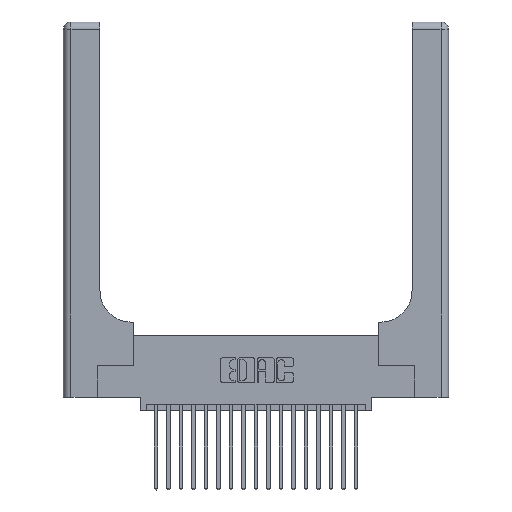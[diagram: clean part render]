
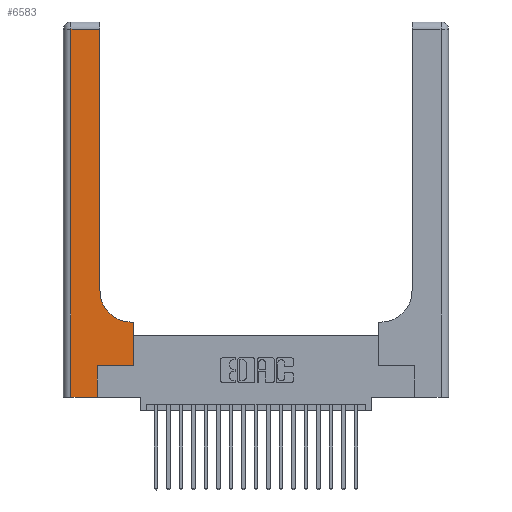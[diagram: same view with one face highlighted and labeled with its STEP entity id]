
A CAD part, top view. The second image highlights one B-rep face of the part: STEP entity #6583.
In plain terms, the highlighted planar face has unit normal (0, 0, 1).
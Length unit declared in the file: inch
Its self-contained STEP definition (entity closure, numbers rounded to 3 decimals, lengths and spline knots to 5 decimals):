
#160 = CARTESIAN_POINT ( 'NONE',  ( 0.06, 2.94, 0.37 ) ) ;
#549 = CARTESIAN_POINT ( 'NONE',  ( 0., 0., 0.37 ) ) ;
#964 = DIRECTION ( 'NONE',  ( 1., 0., 0. ) ) ;
#1575 = LINE ( 'NONE', #14638, #7964 ) ;
#1831 = VERTEX_POINT ( 'NONE', #12233 ) ;
#1888 = LINE ( 'NONE', #549, #21848 ) ;
#2194 = DIRECTION ( 'NONE',  ( 1., 0., 0. ) ) ;
#2305 = DIRECTION ( 'NONE',  ( 0., 1., 0. ) ) ;
#2744 = CARTESIAN_POINT ( 'NONE',  ( 0.5415, 0.85, 0.37 ) ) ;
#3574 = VERTEX_POINT ( 'NONE', #21102 ) ;
#3605 = EDGE_CURVE ( 'NONE', #5653, #17092, #1575, .T. ) ;
#3659 = CIRCLE ( 'NONE', #8920, 0.25 ) ;
#3878 = EDGE_CURVE ( 'NONE', #4522, #4904, #17518, .T. ) ;
#3891 = CARTESIAN_POINT ( 'NONE',  ( 0.2915, 3., 0.37 ) ) ;
#4163 = ORIENTED_EDGE ( 'NONE', *, *, #9384, .T. ) ;
#4275 = CARTESIAN_POINT ( 'NONE',  ( 0.5585, 0.25, 0.37 ) ) ;
#4522 = VERTEX_POINT ( 'NONE', #8512 ) ;
#4691 = VECTOR ( 'NONE', #12994, 39.37008 ) ;
#4701 = VECTOR ( 'NONE', #6234, 39.37008 ) ;
#4904 = VERTEX_POINT ( 'NONE', #16186 ) ;
#5054 = ORIENTED_EDGE ( 'NONE', *, *, #8174, .T. ) ;
#5500 = FACE_OUTER_BOUND ( 'NONE', #9506, .T. ) ;
#5653 = VERTEX_POINT ( 'NONE', #160 ) ;
#5968 = CARTESIAN_POINT ( 'NONE',  ( 0.2915, 0.85, 0.37 ) ) ;
#6234 = DIRECTION ( 'NONE',  ( -1., 0., 0. ) ) ;
#6258 = DIRECTION ( 'NONE',  ( 0., 0., -1. ) ) ;
#6583 = ADVANCED_FACE ( 'NONE', ( #5500 ), #12035, .F. ) ;
#7610 = ORIENTED_EDGE ( 'NONE', *, *, #3878, .T. ) ;
#7964 = VECTOR ( 'NONE', #16348, 39.37008 ) ;
#7982 = VERTEX_POINT ( 'NONE', #11051 ) ;
#8172 = ORIENTED_EDGE ( 'NONE', *, *, #12587, .T. ) ;
#8174 = EDGE_CURVE ( 'NONE', #9683, #1831, #16610, .T. ) ;
#8345 = CARTESIAN_POINT ( 'NONE',  ( 0.06, 0., 0.37 ) ) ;
#8512 = CARTESIAN_POINT ( 'NONE',  ( 0.5585, 0.25, 0.37 ) ) ;
#8640 = ORIENTED_EDGE ( 'NONE', *, *, #20058, .T. ) ;
#8642 = DIRECTION ( 'NONE',  ( 0., 1., 0. ) ) ;
#8920 = AXIS2_PLACEMENT_3D ( 'NONE', #2744, #16185, #964 ) ;
#9384 = EDGE_CURVE ( 'NONE', #20525, #7982, #21616, .T. ) ;
#9411 = DIRECTION ( 'NONE',  ( 1., 0., 0. ) ) ;
#9506 = EDGE_LOOP ( 'NONE', ( #4163, #8640, #14706, #16773, #5054, #18468, #7610, #14855, #8172 ) ) ;
#9532 = CARTESIAN_POINT ( 'NONE',  ( 0., 3., 0.37 ) ) ;
#9611 = CARTESIAN_POINT ( 'NONE',  ( 0.269, 0.25, 0.37 ) ) ;
#9683 = VERTEX_POINT ( 'NONE', #11666 ) ;
#10507 = EDGE_CURVE ( 'NONE', #1831, #4522, #18613, .T. ) ;
#11051 = CARTESIAN_POINT ( 'NONE',  ( 0.2915, 2.94, 0.37 ) ) ;
#11666 = CARTESIAN_POINT ( 'NONE',  ( 0.269, 0., 0.37 ) ) ;
#12035 = PLANE ( 'NONE',  #14204 ) ;
#12233 = CARTESIAN_POINT ( 'NONE',  ( 0.269, 0.25, 0.37 ) ) ;
#12587 = EDGE_CURVE ( 'NONE', #3574, #20525, #3659, .T. ) ;
#12994 = DIRECTION ( 'NONE',  ( -1., 0., 0. ) ) ;
#14066 = EDGE_CURVE ( 'NONE', #4904, #3574, #18217, .T. ) ;
#14204 = AXIS2_PLACEMENT_3D ( 'NONE', #9532, #6258, #16349 ) ;
#14638 = CARTESIAN_POINT ( 'NONE',  ( 0.06, 3., 0.37 ) ) ;
#14706 = ORIENTED_EDGE ( 'NONE', *, *, #3605, .T. ) ;
#14855 = ORIENTED_EDGE ( 'NONE', *, *, #14066, .T. ) ;
#15474 = VECTOR ( 'NONE', #2305, 39.37008 ) ;
#16185 = DIRECTION ( 'NONE',  ( 0., 0., -1. ) ) ;
#16186 = CARTESIAN_POINT ( 'NONE',  ( 0.5585, 0.6, 0.37 ) ) ;
#16348 = DIRECTION ( 'NONE',  ( 0., -1., 0. ) ) ;
#16349 = DIRECTION ( 'NONE',  ( -1., 0., 0. ) ) ;
#16610 = LINE ( 'NONE', #22029, #21397 ) ;
#16613 = EDGE_CURVE ( 'NONE', #17092, #9683, #1888, .T. ) ;
#16773 = ORIENTED_EDGE ( 'NONE', *, *, #16613, .T. ) ;
#17092 = VERTEX_POINT ( 'NONE', #8345 ) ;
#17378 = LINE ( 'NONE', #21201, #4691 ) ;
#17518 = LINE ( 'NONE', #4275, #20982 ) ;
#17754 = DIRECTION ( 'NONE',  ( 0., 1., 0. ) ) ;
#18217 = LINE ( 'NONE', #19662, #4701 ) ;
#18468 = ORIENTED_EDGE ( 'NONE', *, *, #10507, .T. ) ;
#18613 = LINE ( 'NONE', #9611, #19678 ) ;
#19662 = CARTESIAN_POINT ( 'NONE',  ( 0.2915, 0.6, 0.37 ) ) ;
#19678 = VECTOR ( 'NONE', #9411, 39.37008 ) ;
#20058 = EDGE_CURVE ( 'NONE', #7982, #5653, #17378, .T. ) ;
#20525 = VERTEX_POINT ( 'NONE', #5968 ) ;
#20982 = VECTOR ( 'NONE', #17754, 39.37008 ) ;
#21102 = CARTESIAN_POINT ( 'NONE',  ( 0.5415, 0.6, 0.37 ) ) ;
#21201 = CARTESIAN_POINT ( 'NONE',  ( 0., 2.94, 0.37 ) ) ;
#21397 = VECTOR ( 'NONE', #8642, 39.37008 ) ;
#21616 = LINE ( 'NONE', #3891, #15474 ) ;
#21848 = VECTOR ( 'NONE', #2194, 39.37008 ) ;
#22029 = CARTESIAN_POINT ( 'NONE',  ( 0.269, 0., 0.37 ) ) ;
